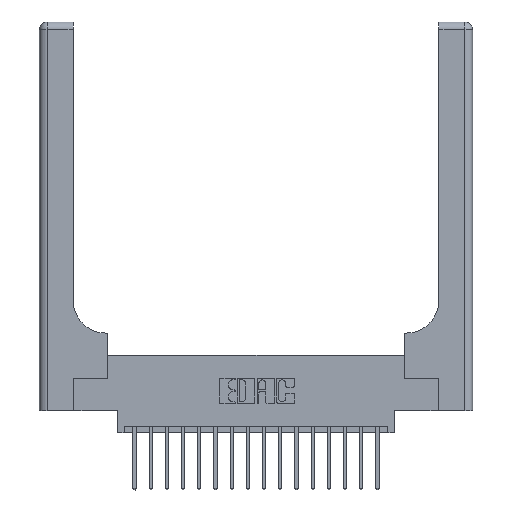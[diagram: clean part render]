
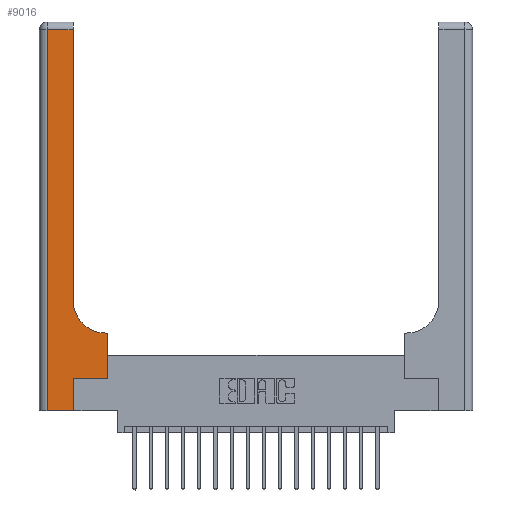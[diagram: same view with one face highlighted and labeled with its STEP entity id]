
A CAD part, top view. The second image highlights one B-rep face of the part: STEP entity #9016.
In plain terms, the highlighted planar face has unit normal (0, 0, 1).
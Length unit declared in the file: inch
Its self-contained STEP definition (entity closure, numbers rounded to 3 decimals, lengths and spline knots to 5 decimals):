
#190 = EDGE_CURVE ( 'NONE', #10814, #18412, #2315, .T. ) ;
#259 = DIRECTION ( 'NONE',  ( 1., 0., 0. ) ) ;
#704 = VERTEX_POINT ( 'NONE', #6171 ) ;
#707 = VERTEX_POINT ( 'NONE', #7664 ) ;
#925 = AXIS2_PLACEMENT_3D ( 'NONE', #15932, #7074, #17401 ) ;
#1379 = EDGE_CURVE ( 'NONE', #17625, #707, #15411, .T. ) ;
#1617 = LINE ( 'NONE', #6664, #9581 ) ;
#1708 = CARTESIAN_POINT ( 'NONE',  ( 0.06, 0., 0.37 ) ) ;
#1728 = CARTESIAN_POINT ( 'NONE',  ( 0.26, 3., 0.37 ) ) ;
#1763 = VECTOR ( 'NONE', #16236, 39.37008 ) ;
#2315 = LINE ( 'NONE', #15448, #9832 ) ;
#2400 = VECTOR ( 'NONE', #7493, 39.37008 ) ;
#3108 = EDGE_LOOP ( 'NONE', ( #8429, #8521, #8651, #8821, #9405, #9730, #9766, #9771, #9985 ) ) ;
#3357 = DIRECTION ( 'NONE',  ( 1., 0., 0. ) ) ;
#3404 = VECTOR ( 'NONE', #3357, 39.37008 ) ;
#3545 = VECTOR ( 'NONE', #259, 39.37008 ) ;
#3724 = VERTEX_POINT ( 'NONE', #17915 ) ;
#3786 = EDGE_CURVE ( 'NONE', #3724, #10814, #4862, .T. ) ;
#3864 = PLANE ( 'NONE',  #19235 ) ;
#4862 = LINE ( 'NONE', #1728, #11843 ) ;
#5157 = EDGE_CURVE ( 'NONE', #15613, #12840, #13638, .T. ) ;
#5183 = EDGE_CURVE ( 'NONE', #15668, #15613, #17111, .T. ) ;
#5314 = EDGE_CURVE ( 'NONE', #704, #15668, #11324, .T. ) ;
#5374 = DIRECTION ( 'NONE',  ( -1., 0., 0. ) ) ;
#6171 = CARTESIAN_POINT ( 'NONE',  ( 0.265, 0.25, 0.37 ) ) ;
#6664 = CARTESIAN_POINT ( 'NONE',  ( 0.265, 0., 0.37 ) ) ;
#7074 = DIRECTION ( 'NONE',  ( 0., 0., -1. ) ) ;
#7075 = FACE_OUTER_BOUND ( 'NONE', #3108, .T. ) ;
#7493 = DIRECTION ( 'NONE',  ( 0., -1., 0. ) ) ;
#7664 = CARTESIAN_POINT ( 'NONE',  ( 0.265, 0., 0.37 ) ) ;
#8342 = CIRCLE ( 'NONE', #925, 0.25 ) ;
#8429 = ORIENTED_EDGE ( 'NONE', *, *, #3786, .T. ) ;
#8521 = ORIENTED_EDGE ( 'NONE', *, *, #190, .T. ) ;
#8651 = ORIENTED_EDGE ( 'NONE', *, *, #14384, .T. ) ;
#8821 = ORIENTED_EDGE ( 'NONE', *, *, #1379, .T. ) ;
#8849 = DIRECTION ( 'NONE',  ( 0., 1., 0. ) ) ;
#9016 = ADVANCED_FACE ( 'NONE', ( #7075 ), #3864, .F. ) ;
#9405 = ORIENTED_EDGE ( 'NONE', *, *, #16616, .T. ) ;
#9581 = VECTOR ( 'NONE', #15537, 39.37008 ) ;
#9599 = CARTESIAN_POINT ( 'NONE',  ( 0.06, 2.94, 0.37 ) ) ;
#9730 = ORIENTED_EDGE ( 'NONE', *, *, #5314, .T. ) ;
#9766 = ORIENTED_EDGE ( 'NONE', *, *, #5183, .T. ) ;
#9771 = ORIENTED_EDGE ( 'NONE', *, *, #5157, .T. ) ;
#9832 = VECTOR ( 'NONE', #13881, 39.37008 ) ;
#9985 = ORIENTED_EDGE ( 'NONE', *, *, #18445, .T. ) ;
#10364 = CARTESIAN_POINT ( 'NONE',  ( 0.528, 0.25, 0.37 ) ) ;
#10765 = CARTESIAN_POINT ( 'NONE',  ( 0., 0., 0.37 ) ) ;
#10814 = VERTEX_POINT ( 'NONE', #13718 ) ;
#11324 = LINE ( 'NONE', #13749, #3404 ) ;
#11843 = VECTOR ( 'NONE', #13639, 39.37008 ) ;
#12840 = VERTEX_POINT ( 'NONE', #12875 ) ;
#12875 = CARTESIAN_POINT ( 'NONE',  ( 0.51, 0.6, 0.37 ) ) ;
#13187 = VECTOR ( 'NONE', #8849, 39.37008 ) ;
#13638 = LINE ( 'NONE', #17639, #1763 ) ;
#13639 = DIRECTION ( 'NONE',  ( 0., 1., 0. ) ) ;
#13718 = CARTESIAN_POINT ( 'NONE',  ( 0.26, 2.94, 0.37 ) ) ;
#13749 = CARTESIAN_POINT ( 'NONE',  ( 0.265, 0.25, 0.37 ) ) ;
#13881 = DIRECTION ( 'NONE',  ( -1., 0., 0. ) ) ;
#14268 = DIRECTION ( 'NONE',  ( 0., 0., -1. ) ) ;
#14384 = EDGE_CURVE ( 'NONE', #18412, #17625, #17743, .T. ) ;
#15411 = LINE ( 'NONE', #10765, #3545 ) ;
#15448 = CARTESIAN_POINT ( 'NONE',  ( 0., 2.94, 0.37 ) ) ;
#15537 = DIRECTION ( 'NONE',  ( 0., 1., 0. ) ) ;
#15613 = VERTEX_POINT ( 'NONE', #17852 ) ;
#15668 = VERTEX_POINT ( 'NONE', #16517 ) ;
#15692 = CARTESIAN_POINT ( 'NONE',  ( 0., 3., 0.37 ) ) ;
#15932 = CARTESIAN_POINT ( 'NONE',  ( 0.51, 0.85, 0.37 ) ) ;
#16236 = DIRECTION ( 'NONE',  ( -1., 0., 0. ) ) ;
#16517 = CARTESIAN_POINT ( 'NONE',  ( 0.528, 0.25, 0.37 ) ) ;
#16616 = EDGE_CURVE ( 'NONE', #707, #704, #1617, .T. ) ;
#17111 = LINE ( 'NONE', #10364, #13187 ) ;
#17401 = DIRECTION ( 'NONE',  ( 1., 0., 0. ) ) ;
#17625 = VERTEX_POINT ( 'NONE', #1708 ) ;
#17639 = CARTESIAN_POINT ( 'NONE',  ( 0.26, 0.6, 0.37 ) ) ;
#17743 = LINE ( 'NONE', #17820, #2400 ) ;
#17820 = CARTESIAN_POINT ( 'NONE',  ( 0.06, 3., 0.37 ) ) ;
#17852 = CARTESIAN_POINT ( 'NONE',  ( 0.528, 0.6, 0.37 ) ) ;
#17915 = CARTESIAN_POINT ( 'NONE',  ( 0.26, 0.85, 0.37 ) ) ;
#18412 = VERTEX_POINT ( 'NONE', #9599 ) ;
#18445 = EDGE_CURVE ( 'NONE', #12840, #3724, #8342, .T. ) ;
#19235 = AXIS2_PLACEMENT_3D ( 'NONE', #15692, #14268, #5374 ) ;
